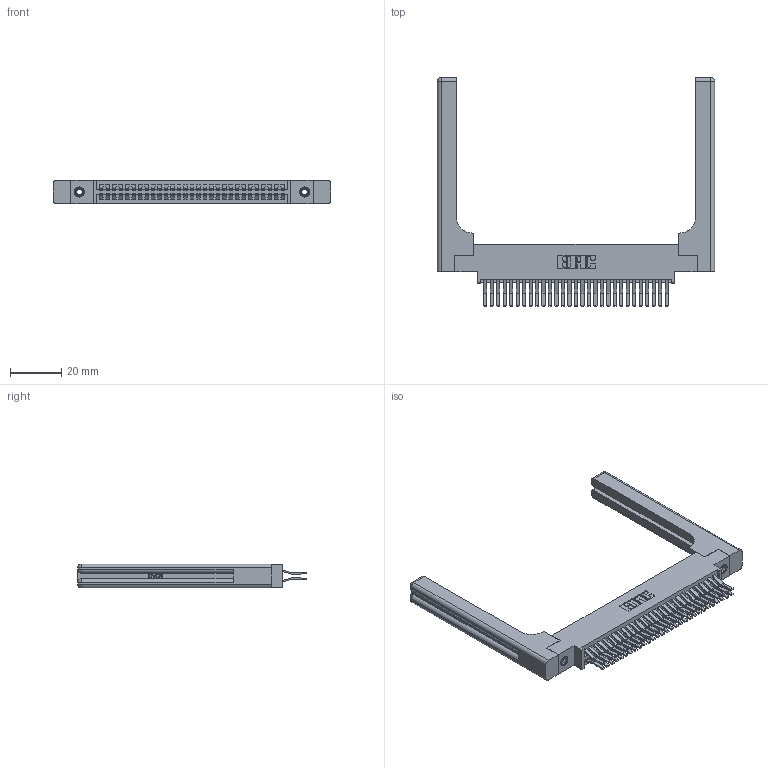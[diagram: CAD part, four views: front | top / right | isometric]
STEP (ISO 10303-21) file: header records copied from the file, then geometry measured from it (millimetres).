
FILE_DESCRIPTION (( 'STEP AP203' ), '1' );
FILE_NAME ('345-058-560-858.STEP', '2019-10-30T06:47:38', ( '' ), ( '' ), 'SwSTEP 2.0', 'SolidWorks 2016', '' );
FILE_SCHEMA (( 'CONFIG_CONTROL_DESIGN' ));
Length unit declared in the file: inch
Products named in the file (5): 345-058-560-858; 345-220-058_345-220-058; 345 Part_0.170 Offset - 0.156 Dia-TH; 345-292-001_560 Tail; 345-250-001_345-250-001-102
Assembly tree (63 placements, depth 2):
  345-058-560-858
    345 Part_0.170 Offset - 0.156 Dia-TH
    345-292-001_560 Tail  x58
    345-250-001_345-250-001-102  x2
    345-220-058_345-220-058  x2
Bounding box: 108.69 x 89.72 x 9.4 mm (x, y, z)
Volume: 19179.2 mm3; surface area: 21750.7 mm2
Topology: 63 solids, 63 shells, 3402 faces, 10009 edges, 6574 vertices
Faces by surface type: plane 2146, cylinder 1196, bspline 36, cone 12, sphere 8, torus 4
Entity records: 29906 total; most frequent: CARTESIAN_POINT 6021, ORIENTED_EDGE 4752, DIRECTION 4260, EDGE_CURVE 2376, VECTOR 2032, LINE 2032, VERTEX_POINT 1574, AXIS2_PLACEMENT_3D 1114
